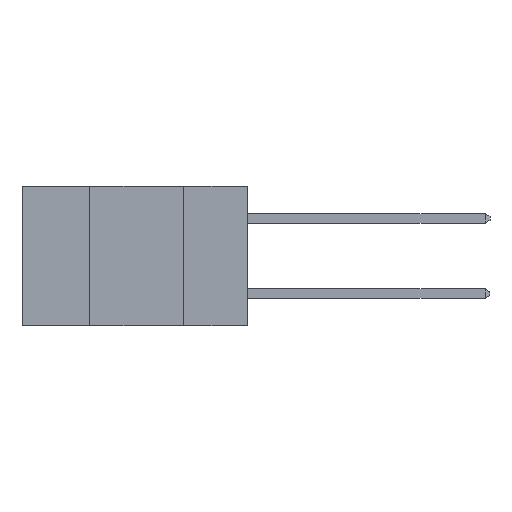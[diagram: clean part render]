
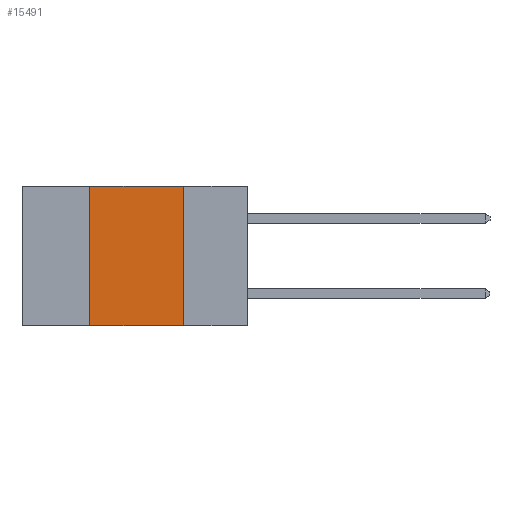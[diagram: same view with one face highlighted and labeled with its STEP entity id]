
A CAD part, left-side view. The second image highlights one B-rep face of the part: STEP entity #15491.
In plain terms, the highlighted planar face has unit normal (-1, 0, 0).
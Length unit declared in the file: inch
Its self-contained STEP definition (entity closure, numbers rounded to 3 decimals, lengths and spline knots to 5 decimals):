
#719 = ORIENTED_EDGE ( 'NONE', *, *, #10546, .T. ) ;
#1610 = CARTESIAN_POINT ( 'NONE',  ( 0., 0.6, 0. ) ) ;
#2284 = EDGE_LOOP ( 'NONE', ( #2677, #4052, #6577, #719 ) ) ;
#2677 = ORIENTED_EDGE ( 'NONE', *, *, #9719, .F. ) ;
#2741 = VECTOR ( 'NONE', #17524, 39.37008 ) ;
#2895 = VECTOR ( 'NONE', #13685, 39.37008 ) ;
#3062 = DIRECTION ( 'NONE',  ( 1., 0., 0. ) ) ;
#3823 = VERTEX_POINT ( 'NONE', #7815 ) ;
#3963 = FACE_OUTER_BOUND ( 'NONE', #2284, .T. ) ;
#4052 = ORIENTED_EDGE ( 'NONE', *, *, #7130, .F. ) ;
#6577 = ORIENTED_EDGE ( 'NONE', *, *, #9833, .F. ) ;
#7010 = AXIS2_PLACEMENT_3D ( 'NONE', #1610, #3062, #13151 ) ;
#7088 = VERTEX_POINT ( 'NONE', #10524 ) ;
#7130 = EDGE_CURVE ( 'NONE', #7088, #14298, #7506, .T. ) ;
#7506 = LINE ( 'NONE', #9140, #2741 ) ;
#7815 = CARTESIAN_POINT ( 'NONE',  ( 0., 0.17, -0.37 ) ) ;
#7951 = VERTEX_POINT ( 'NONE', #13735 ) ;
#8269 = VECTOR ( 'NONE', #16479, 39.37008 ) ;
#8632 = CARTESIAN_POINT ( 'NONE',  ( 0., 0.17, 0. ) ) ;
#9035 = LINE ( 'NONE', #9189, #12828 ) ;
#9140 = CARTESIAN_POINT ( 'NONE',  ( 0., 0.6, 0. ) ) ;
#9189 = CARTESIAN_POINT ( 'NONE',  ( 0., 0.17, 0. ) ) ;
#9719 = EDGE_CURVE ( 'NONE', #14298, #3823, #9035, .T. ) ;
#9833 = EDGE_CURVE ( 'NONE', #7951, #7088, #14374, .T. ) ;
#10272 = PLANE ( 'NONE',  #7010 ) ;
#10524 = CARTESIAN_POINT ( 'NONE',  ( 0., 0.42, 0. ) ) ;
#10546 = EDGE_CURVE ( 'NONE', #7951, #3823, #16216, .T. ) ;
#10623 = DIRECTION ( 'NONE',  ( 0., 0., -1. ) ) ;
#12828 = VECTOR ( 'NONE', #10623, 39.37008 ) ;
#13151 = DIRECTION ( 'NONE',  ( 0., 0., -1. ) ) ;
#13685 = DIRECTION ( 'NONE',  ( 0., 0., 1. ) ) ;
#13735 = CARTESIAN_POINT ( 'NONE',  ( 0., 0.42, -0.37 ) ) ;
#14298 = VERTEX_POINT ( 'NONE', #8632 ) ;
#14374 = LINE ( 'NONE', #16437, #2895 ) ;
#15113 = CARTESIAN_POINT ( 'NONE',  ( 0., 0.6, -0.37 ) ) ;
#15491 = ADVANCED_FACE ( 'NONE', ( #3963 ), #10272, .F. ) ;
#16216 = LINE ( 'NONE', #15113, #8269 ) ;
#16437 = CARTESIAN_POINT ( 'NONE',  ( 0., 0.42, 0. ) ) ;
#16479 = DIRECTION ( 'NONE',  ( 0., -1., 0. ) ) ;
#17524 = DIRECTION ( 'NONE',  ( 0., -1., 0. ) ) ;
